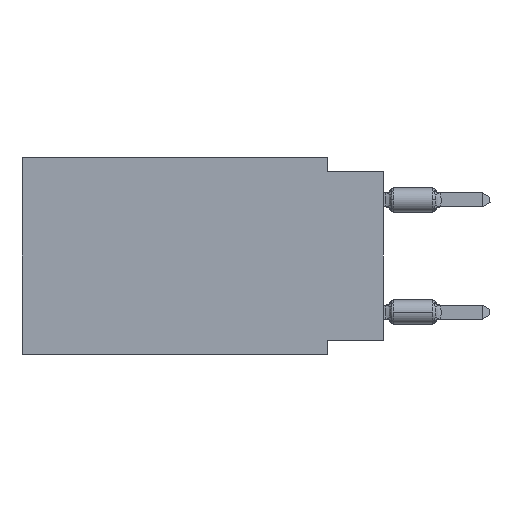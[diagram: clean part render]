
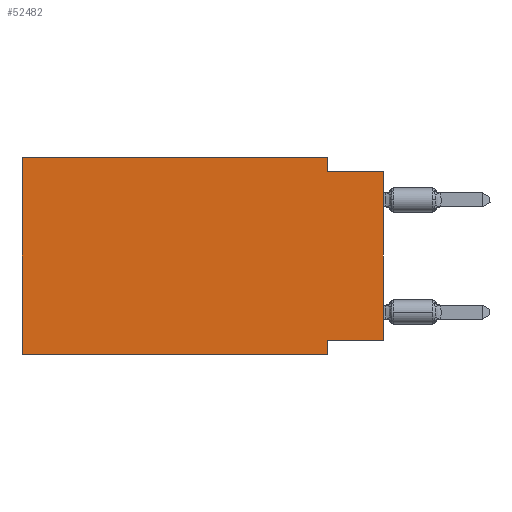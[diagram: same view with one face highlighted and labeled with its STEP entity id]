
A CAD part, left-side view. The second image highlights one B-rep face of the part: STEP entity #52482.
In plain terms, the highlighted planar face has unit normal (-1, 0, 0).
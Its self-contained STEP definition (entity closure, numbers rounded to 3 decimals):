
#1014 = DIRECTION ( 'NONE',  ( 0., -1., 0. ) ) ;
#2314 = VERTEX_POINT ( 'NONE', #40759 ) ;
#3768 = CARTESIAN_POINT ( 'NONE',  ( 0., 2.54, -8.255 ) ) ;
#3940 = CARTESIAN_POINT ( 'NONE',  ( 0., 0., -8.255 ) ) ;
#4413 = AXIS2_PLACEMENT_3D ( 'NONE', #9447, #42151, #57182 ) ;
#5113 = EDGE_CURVE ( 'NONE', #63454, #2314, #14173, .T. ) ;
#5817 = CARTESIAN_POINT ( 'NONE',  ( 0., 0., -0.635 ) ) ;
#7272 = EDGE_CURVE ( 'NONE', #45220, #63454, #15226, .T. ) ;
#7622 = LINE ( 'NONE', #5817, #39430 ) ;
#7715 = VECTOR ( 'NONE', #61829, 1000. ) ;
#8266 = VECTOR ( 'NONE', #43795, 1000. ) ;
#9278 = CARTESIAN_POINT ( 'NONE',  ( 0., 2.54, -8.89 ) ) ;
#9447 = CARTESIAN_POINT ( 'NONE',  ( 0., 16.383, 0. ) ) ;
#9785 = CARTESIAN_POINT ( 'NONE',  ( 0., 0., -0.635 ) ) ;
#11512 = VECTOR ( 'NONE', #19506, 1000. ) ;
#11705 = VECTOR ( 'NONE', #43188, 1000. ) ;
#13009 = ORIENTED_EDGE ( 'NONE', *, *, #5113, .F. ) ;
#13429 = EDGE_CURVE ( 'NONE', #45220, #45202, #44623, .T. ) ;
#13554 = ORIENTED_EDGE ( 'NONE', *, *, #34395, .F. ) ;
#14106 = ORIENTED_EDGE ( 'NONE', *, *, #64051, .F. ) ;
#14173 = LINE ( 'NONE', #9278, #11705 ) ;
#14769 = EDGE_CURVE ( 'NONE', #64424, #2314, #20269, .T. ) ;
#15226 = LINE ( 'NONE', #25666, #7715 ) ;
#19506 = DIRECTION ( 'NONE',  ( 0., 0., 1. ) ) ;
#19580 = CARTESIAN_POINT ( 'NONE',  ( 0., 2.54, 0. ) ) ;
#20269 = LINE ( 'NONE', #60065, #47056 ) ;
#22662 = CARTESIAN_POINT ( 'NONE',  ( 0., 16.383, 0. ) ) ;
#23205 = ORIENTED_EDGE ( 'NONE', *, *, #7272, .F. ) ;
#23420 = EDGE_CURVE ( 'NONE', #41801, #45202, #7622, .T. ) ;
#23643 = EDGE_LOOP ( 'NONE', ( #50691, #58234, #40388, #14106, #13554, #60393, #13009, #23205 ) ) ;
#23920 = CARTESIAN_POINT ( 'NONE',  ( 0., 16.383, 0. ) ) ;
#25666 = CARTESIAN_POINT ( 'NONE',  ( 0., 0., -8.255 ) ) ;
#25825 = EDGE_CURVE ( 'NONE', #56441, #41801, #43900, .T. ) ;
#26912 = DIRECTION ( 'NONE',  ( 0., -1., 0. ) ) ;
#27160 = CARTESIAN_POINT ( 'NONE',  ( 0., 16.383, -8.89 ) ) ;
#28646 = CARTESIAN_POINT ( 'NONE',  ( 0., 2.54, -0.635 ) ) ;
#30351 = VECTOR ( 'NONE', #42215, 1000. ) ;
#32990 = CARTESIAN_POINT ( 'NONE',  ( 0., 16.383, 0. ) ) ;
#34395 = EDGE_CURVE ( 'NONE', #64424, #37620, #64355, .T. ) ;
#34560 = FACE_OUTER_BOUND ( 'NONE', #23643, .T. ) ;
#37620 = VERTEX_POINT ( 'NONE', #32990 ) ;
#39002 = DIRECTION ( 'NONE',  ( 0., 0., -1. ) ) ;
#39430 = VECTOR ( 'NONE', #26912, 1000. ) ;
#40388 = ORIENTED_EDGE ( 'NONE', *, *, #25825, .F. ) ;
#40759 = CARTESIAN_POINT ( 'NONE',  ( 0., 2.54, -8.89 ) ) ;
#41801 = VERTEX_POINT ( 'NONE', #28646 ) ;
#42151 = DIRECTION ( 'NONE',  ( 1., 0., 0. ) ) ;
#42215 = DIRECTION ( 'NONE',  ( 0., -1., 0. ) ) ;
#43188 = DIRECTION ( 'NONE',  ( 0., 0., -1. ) ) ;
#43795 = DIRECTION ( 'NONE',  ( 0., 0., 1. ) ) ;
#43900 = LINE ( 'NONE', #63812, #61298 ) ;
#44623 = LINE ( 'NONE', #59952, #11512 ) ;
#45202 = VERTEX_POINT ( 'NONE', #9785 ) ;
#45220 = VERTEX_POINT ( 'NONE', #3940 ) ;
#47056 = VECTOR ( 'NONE', #1014, 1000. ) ;
#48084 = LINE ( 'NONE', #22662, #30351 ) ;
#50691 = ORIENTED_EDGE ( 'NONE', *, *, #13429, .T. ) ;
#52482 = ADVANCED_FACE ( 'NONE', ( #34560 ), #63935, .F. ) ;
#56441 = VERTEX_POINT ( 'NONE', #19580 ) ;
#57182 = DIRECTION ( 'NONE',  ( 0., 0., -1. ) ) ;
#58234 = ORIENTED_EDGE ( 'NONE', *, *, #23420, .F. ) ;
#59952 = CARTESIAN_POINT ( 'NONE',  ( 0., 0., 0. ) ) ;
#60065 = CARTESIAN_POINT ( 'NONE',  ( 0., 16.383, -8.89 ) ) ;
#60393 = ORIENTED_EDGE ( 'NONE', *, *, #14769, .T. ) ;
#61298 = VECTOR ( 'NONE', #39002, 1000. ) ;
#61829 = DIRECTION ( 'NONE',  ( 0., 1., 0. ) ) ;
#63454 = VERTEX_POINT ( 'NONE', #3768 ) ;
#63812 = CARTESIAN_POINT ( 'NONE',  ( 0., 2.54, 0. ) ) ;
#63935 = PLANE ( 'NONE',  #4413 ) ;
#64051 = EDGE_CURVE ( 'NONE', #37620, #56441, #48084, .T. ) ;
#64355 = LINE ( 'NONE', #23920, #8266 ) ;
#64424 = VERTEX_POINT ( 'NONE', #27160 ) ;
